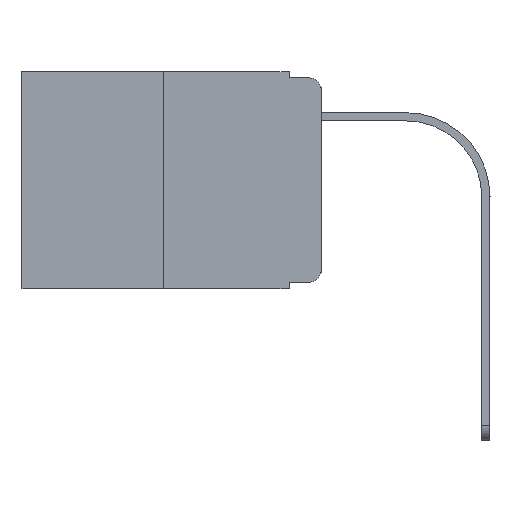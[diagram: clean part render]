
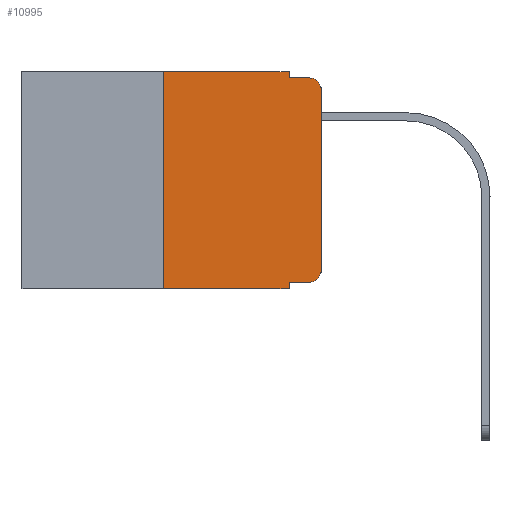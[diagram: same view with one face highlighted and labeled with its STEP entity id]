
A CAD part, left-side view. The second image highlights one B-rep face of the part: STEP entity #10995.
In plain terms, the highlighted planar face has unit normal (-1, 0, 0).
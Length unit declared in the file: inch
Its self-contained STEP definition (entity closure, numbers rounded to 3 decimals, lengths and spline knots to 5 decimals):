
#174 = LINE ( 'NONE', #5555, #12268 ) ;
#255 = CARTESIAN_POINT ( 'NONE',  ( 0., 0.051, -0.333 ) ) ;
#389 = LINE ( 'NONE', #11442, #2869 ) ;
#505 = EDGE_CURVE ( 'NONE', #9569, #8745, #14218, .T. ) ;
#751 = CARTESIAN_POINT ( 'NONE',  ( 0., 0.051, 0. ) ) ;
#1042 = VERTEX_POINT ( 'NONE', #751 ) ;
#1052 = VERTEX_POINT ( 'NONE', #12334 ) ;
#1063 = CIRCLE ( 'NONE', #9561, 0.02 ) ;
#1180 = DIRECTION ( 'NONE',  ( 1., 0., 0. ) ) ;
#1185 = CARTESIAN_POINT ( 'NONE',  ( 0., 0., -0.313 ) ) ;
#1703 = CARTESIAN_POINT ( 'NONE',  ( 0., 0.051, 0. ) ) ;
#1782 = CARTESIAN_POINT ( 'NONE',  ( 0., 0.051, -0.01 ) ) ;
#1945 = CARTESIAN_POINT ( 'NONE',  ( 0., 0.051, -0.343 ) ) ;
#2273 = VECTOR ( 'NONE', #7296, 39.37008 ) ;
#2357 = ORIENTED_EDGE ( 'NONE', *, *, #12695, .T. ) ;
#2418 = EDGE_CURVE ( 'NONE', #4088, #9569, #389, .T. ) ;
#2454 = LINE ( 'NONE', #8142, #6713 ) ;
#2790 = AXIS2_PLACEMENT_3D ( 'NONE', #12696, #15472, #5879 ) ;
#2869 = VECTOR ( 'NONE', #10331, 39.37008 ) ;
#2941 = EDGE_CURVE ( 'NONE', #1052, #15834, #4133, .T. ) ;
#3984 = ORIENTED_EDGE ( 'NONE', *, *, #14429, .F. ) ;
#3988 = CARTESIAN_POINT ( 'NONE',  ( 0., 0., -0.03 ) ) ;
#4088 = VERTEX_POINT ( 'NONE', #1185 ) ;
#4104 = ORIENTED_EDGE ( 'NONE', *, *, #5576, .F. ) ;
#4107 = DIRECTION ( 'NONE',  ( 0., 0., -1. ) ) ;
#4133 = LINE ( 'NONE', #9733, #6869 ) ;
#4222 = AXIS2_PLACEMENT_3D ( 'NONE', #16748, #1180, #4107 ) ;
#4328 = ORIENTED_EDGE ( 'NONE', *, *, #2418, .T. ) ;
#4715 = LINE ( 'NONE', #13193, #7042 ) ;
#4718 = ORIENTED_EDGE ( 'NONE', *, *, #5420, .T. ) ;
#4962 = DIRECTION ( 'NONE',  ( 0., 0., 1. ) ) ;
#5420 = EDGE_CURVE ( 'NONE', #6074, #9719, #17622, .T. ) ;
#5555 = CARTESIAN_POINT ( 'NONE',  ( 0., 0.051, 0. ) ) ;
#5576 = EDGE_CURVE ( 'NONE', #9828, #8745, #2454, .T. ) ;
#5658 = DIRECTION ( 'NONE',  ( -1., 0., 0. ) ) ;
#5769 = ORIENTED_EDGE ( 'NONE', *, *, #15266, .F. ) ;
#5867 = DIRECTION ( 'NONE',  ( 0., -1., 0. ) ) ;
#5879 = DIRECTION ( 'NONE',  ( 0., 0., -1. ) ) ;
#6074 = VERTEX_POINT ( 'NONE', #255 ) ;
#6713 = VECTOR ( 'NONE', #13775, 39.37008 ) ;
#6869 = VECTOR ( 'NONE', #5867, 39.37008 ) ;
#6950 = PLANE ( 'NONE',  #4222 ) ;
#7042 = VECTOR ( 'NONE', #11791, 39.37008 ) ;
#7196 = CARTESIAN_POINT ( 'NONE',  ( 0., 0.02, -0.313 ) ) ;
#7288 = DIRECTION ( 'NONE',  ( 0., 0., -1. ) ) ;
#7296 = DIRECTION ( 'NONE',  ( 0., 0., -1. ) ) ;
#7807 = LINE ( 'NONE', #14812, #9729 ) ;
#7921 = CARTESIAN_POINT ( 'NONE',  ( 0., 0.051, -0.333 ) ) ;
#7979 = EDGE_CURVE ( 'NONE', #1052, #17677, #7807, .T. ) ;
#8142 = CARTESIAN_POINT ( 'NONE',  ( 0., 0.051, -0.01 ) ) ;
#8745 = VERTEX_POINT ( 'NONE', #15561 ) ;
#9561 = AXIS2_PLACEMENT_3D ( 'NONE', #7196, #5658, #7288 ) ;
#9569 = VERTEX_POINT ( 'NONE', #3988 ) ;
#9719 = VERTEX_POINT ( 'NONE', #11979 ) ;
#9729 = VECTOR ( 'NONE', #4962, 39.37008 ) ;
#9733 = CARTESIAN_POINT ( 'NONE',  ( 0., 0.473, -0.343 ) ) ;
#9828 = VERTEX_POINT ( 'NONE', #1782 ) ;
#10331 = DIRECTION ( 'NONE',  ( 0., 0., 1. ) ) ;
#10995 = ADVANCED_FACE ( 'NONE', ( #11096 ), #6950, .F. ) ;
#11096 = FACE_OUTER_BOUND ( 'NONE', #11768, .T. ) ;
#11442 = CARTESIAN_POINT ( 'NONE',  ( 0., 0., 0. ) ) ;
#11726 = ORIENTED_EDGE ( 'NONE', *, *, #2941, .T. ) ;
#11768 = EDGE_LOOP ( 'NONE', ( #4328, #14502, #4104, #3984, #14252, #16055, #11726, #5769, #4718, #2357 ) ) ;
#11791 = DIRECTION ( 'NONE',  ( 0., -1., 0. ) ) ;
#11979 = CARTESIAN_POINT ( 'NONE',  ( 0., 0.02, -0.333 ) ) ;
#12268 = VECTOR ( 'NONE', #18177, 39.37008 ) ;
#12334 = CARTESIAN_POINT ( 'NONE',  ( 0., 0.25, -0.343 ) ) ;
#12695 = EDGE_CURVE ( 'NONE', #9719, #4088, #1063, .T. ) ;
#12696 = CARTESIAN_POINT ( 'NONE',  ( 0., 0.02, -0.03 ) ) ;
#13193 = CARTESIAN_POINT ( 'NONE',  ( 0., 0.473, 0. ) ) ;
#13546 = DIRECTION ( 'NONE',  ( 0., -1., 0. ) ) ;
#13775 = DIRECTION ( 'NONE',  ( 0., -1., 0. ) ) ;
#14218 = CIRCLE ( 'NONE', #2790, 0.02 ) ;
#14252 = ORIENTED_EDGE ( 'NONE', *, *, #17279, .F. ) ;
#14429 = EDGE_CURVE ( 'NONE', #1042, #9828, #174, .T. ) ;
#14502 = ORIENTED_EDGE ( 'NONE', *, *, #505, .T. ) ;
#14812 = CARTESIAN_POINT ( 'NONE',  ( 0., 0.25, 0. ) ) ;
#15266 = EDGE_CURVE ( 'NONE', #6074, #15834, #17263, .T. ) ;
#15472 = DIRECTION ( 'NONE',  ( -1., 0., 0. ) ) ;
#15532 = VECTOR ( 'NONE', #13546, 39.37008 ) ;
#15561 = CARTESIAN_POINT ( 'NONE',  ( 0., 0.02, -0.01 ) ) ;
#15834 = VERTEX_POINT ( 'NONE', #1945 ) ;
#16055 = ORIENTED_EDGE ( 'NONE', *, *, #7979, .F. ) ;
#16748 = CARTESIAN_POINT ( 'NONE',  ( 0., 0.473, 0. ) ) ;
#17263 = LINE ( 'NONE', #1703, #2273 ) ;
#17279 = EDGE_CURVE ( 'NONE', #17677, #1042, #4715, .T. ) ;
#17500 = CARTESIAN_POINT ( 'NONE',  ( 0., 0.25, 0. ) ) ;
#17622 = LINE ( 'NONE', #7921, #15532 ) ;
#17677 = VERTEX_POINT ( 'NONE', #17500 ) ;
#18177 = DIRECTION ( 'NONE',  ( 0., 0., -1. ) ) ;
